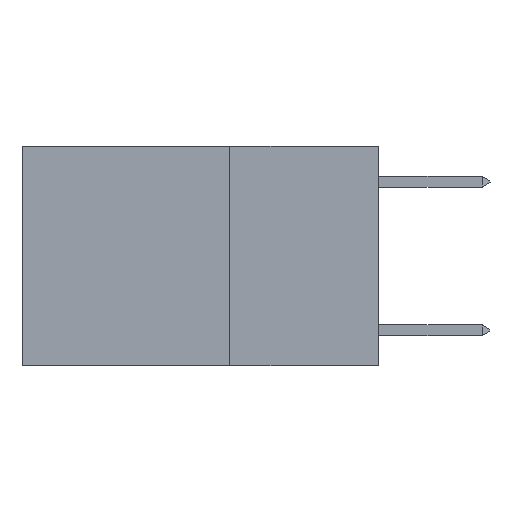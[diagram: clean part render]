
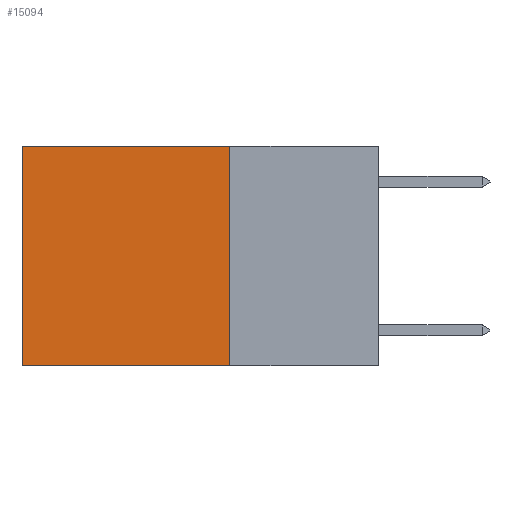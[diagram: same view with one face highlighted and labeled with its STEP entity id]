
A CAD part, left-side view. The second image highlights one B-rep face of the part: STEP entity #15094.
In plain terms, the highlighted planar face has unit normal (-1, 0, 0).
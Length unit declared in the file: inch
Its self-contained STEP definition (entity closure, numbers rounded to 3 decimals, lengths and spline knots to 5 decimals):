
#162 = FACE_OUTER_BOUND ( 'NONE', #2020, .T. ) ;
#598 = VERTEX_POINT ( 'NONE', #12495 ) ;
#1107 = EDGE_CURVE ( 'NONE', #12024, #1405, #6686, .T. ) ;
#1405 = VERTEX_POINT ( 'NONE', #6883 ) ;
#2020 = EDGE_LOOP ( 'NONE', ( #5878, #5985, #6068, #6081 ) ) ;
#2093 = CARTESIAN_POINT ( 'NONE',  ( 0.2625, 0.25, 0. ) ) ;
#2826 = LINE ( 'NONE', #12497, #8760 ) ;
#3440 = VECTOR ( 'NONE', #10725, 39.37008 ) ;
#4203 = LINE ( 'NONE', #7113, #9939 ) ;
#4672 = DIRECTION ( 'NONE',  ( 0., 0., -1. ) ) ;
#4751 = CARTESIAN_POINT ( 'NONE',  ( 0.2625, 0.25, -0.37 ) ) ;
#5192 = EDGE_CURVE ( 'NONE', #598, #12024, #10403, .T. ) ;
#5878 = ORIENTED_EDGE ( 'NONE', *, *, #8796, .T. ) ;
#5985 = ORIENTED_EDGE ( 'NONE', *, *, #1107, .F. ) ;
#6068 = ORIENTED_EDGE ( 'NONE', *, *, #5192, .F. ) ;
#6081 = ORIENTED_EDGE ( 'NONE', *, *, #8076, .T. ) ;
#6686 = LINE ( 'NONE', #10962, #3440 ) ;
#6883 = CARTESIAN_POINT ( 'NONE',  ( 0.2625, 0.6, -0.37 ) ) ;
#6984 = AXIS2_PLACEMENT_3D ( 'NONE', #2093, #11493, #4672 ) ;
#7113 = CARTESIAN_POINT ( 'NONE',  ( 0.2625, 0.6, 0. ) ) ;
#7434 = VECTOR ( 'NONE', #14369, 39.37008 ) ;
#8061 = DIRECTION ( 'NONE',  ( 0., 1., 0. ) ) ;
#8076 = EDGE_CURVE ( 'NONE', #598, #11935, #2826, .T. ) ;
#8241 = DIRECTION ( 'NONE',  ( 0., 0., -1. ) ) ;
#8760 = VECTOR ( 'NONE', #8061, 39.37008 ) ;
#8796 = EDGE_CURVE ( 'NONE', #11935, #1405, #4203, .T. ) ;
#9939 = VECTOR ( 'NONE', #8241, 39.37008 ) ;
#10255 = CARTESIAN_POINT ( 'NONE',  ( 0.2625, 0.6, 0. ) ) ;
#10333 = PLANE ( 'NONE',  #6984 ) ;
#10403 = LINE ( 'NONE', #13261, #7434 ) ;
#10725 = DIRECTION ( 'NONE',  ( 0., 1., 0. ) ) ;
#10962 = CARTESIAN_POINT ( 'NONE',  ( 0.2625, 0.25, -0.37 ) ) ;
#11493 = DIRECTION ( 'NONE',  ( 1., 0., 0. ) ) ;
#11935 = VERTEX_POINT ( 'NONE', #10255 ) ;
#12024 = VERTEX_POINT ( 'NONE', #4751 ) ;
#12495 = CARTESIAN_POINT ( 'NONE',  ( 0.2625, 0.25, 0. ) ) ;
#12497 = CARTESIAN_POINT ( 'NONE',  ( 0.2625, 0.25, 0. ) ) ;
#13261 = CARTESIAN_POINT ( 'NONE',  ( 0.2625, 0.25, 0. ) ) ;
#14369 = DIRECTION ( 'NONE',  ( 0., 0., -1. ) ) ;
#15094 = ADVANCED_FACE ( 'NONE', ( #162 ), #10333, .F. ) ;
